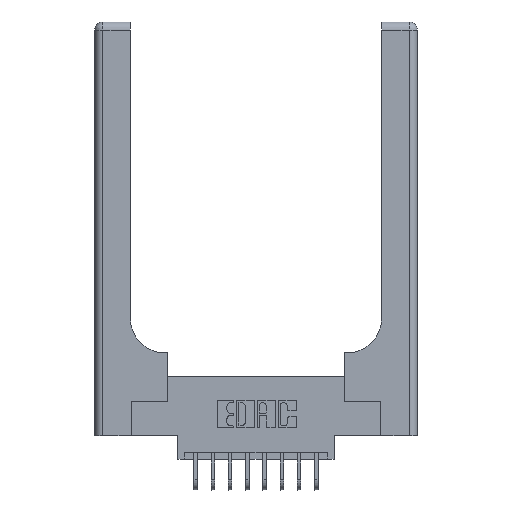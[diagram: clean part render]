
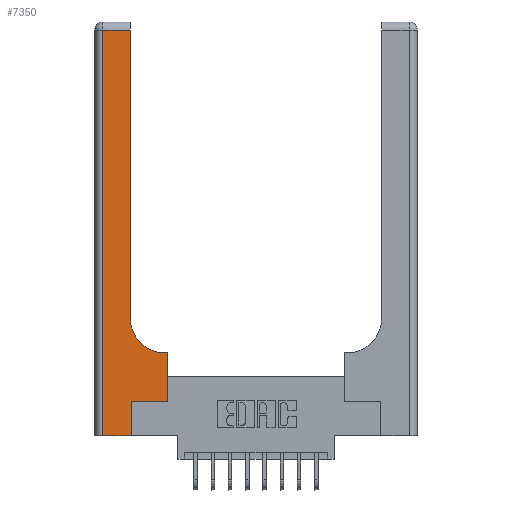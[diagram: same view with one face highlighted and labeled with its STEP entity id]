
A CAD part, top view. The second image highlights one B-rep face of the part: STEP entity #7350.
In plain terms, the highlighted planar face has unit normal (0, 0, 1).
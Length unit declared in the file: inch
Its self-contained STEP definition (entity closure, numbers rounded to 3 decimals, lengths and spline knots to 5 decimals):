
#139 = AXIS2_PLACEMENT_3D ( 'NONE', #10508, #4011, #13096 ) ;
#195 = LINE ( 'NONE', #4476, #13621 ) ;
#412 = CARTESIAN_POINT ( 'NONE',  ( 0.06, 3., 0.37 ) ) ;
#425 = ORIENTED_EDGE ( 'NONE', *, *, #13636, .T. ) ;
#870 = VECTOR ( 'NONE', #14672, 39.37008 ) ;
#946 = EDGE_CURVE ( 'NONE', #8027, #1399, #11583, .T. ) ;
#1140 = LINE ( 'NONE', #3094, #14382 ) ;
#1165 = CARTESIAN_POINT ( 'NONE',  ( 0.528, 0.25, 0.37 ) ) ;
#1182 = LINE ( 'NONE', #11846, #6109 ) ;
#1399 = VERTEX_POINT ( 'NONE', #14394 ) ;
#1741 = EDGE_CURVE ( 'NONE', #9085, #14748, #13734, .T. ) ;
#1754 = ORIENTED_EDGE ( 'NONE', *, *, #1741, .T. ) ;
#2352 = CARTESIAN_POINT ( 'NONE',  ( 0.528, 0.6, 0.37 ) ) ;
#2719 = PLANE ( 'NONE',  #139 ) ;
#2959 = CARTESIAN_POINT ( 'NONE',  ( 0.06, 2.94, 0.37 ) ) ;
#2977 = DIRECTION ( 'NONE',  ( -1., 0., 0. ) ) ;
#3094 = CARTESIAN_POINT ( 'NONE',  ( 0.26, 0.6, 0.37 ) ) ;
#3334 = ORIENTED_EDGE ( 'NONE', *, *, #13177, .T. ) ;
#3459 = CARTESIAN_POINT ( 'NONE',  ( 0.265, 0., 0.37 ) ) ;
#3474 = VERTEX_POINT ( 'NONE', #2959 ) ;
#3480 = EDGE_LOOP ( 'NONE', ( #13267, #8925, #3334, #16211, #7338, #14105, #1754, #425, #15475 ) ) ;
#3570 = CARTESIAN_POINT ( 'NONE',  ( 0.265, 0.25, 0.37 ) ) ;
#3919 = AXIS2_PLACEMENT_3D ( 'NONE', #12390, #7409, #16470 ) ;
#3924 = EDGE_CURVE ( 'NONE', #4167, #8027, #4488, .T. ) ;
#4011 = DIRECTION ( 'NONE',  ( 0., 0., -1. ) ) ;
#4067 = DIRECTION ( 'NONE',  ( 0., 1., 0. ) ) ;
#4167 = VERTEX_POINT ( 'NONE', #5222 ) ;
#4476 = CARTESIAN_POINT ( 'NONE',  ( 0., 2.94, 0.37 ) ) ;
#4488 = CIRCLE ( 'NONE', #3919, 0.25 ) ;
#4584 = VECTOR ( 'NONE', #5874, 39.37008 ) ;
#4842 = LINE ( 'NONE', #412, #16899 ) ;
#5222 = CARTESIAN_POINT ( 'NONE',  ( 0.51, 0.6, 0.37 ) ) ;
#5644 = DIRECTION ( 'NONE',  ( 0., -1., 0. ) ) ;
#5874 = DIRECTION ( 'NONE',  ( 1., 0., 0. ) ) ;
#6109 = VECTOR ( 'NONE', #4067, 39.37008 ) ;
#6215 = DIRECTION ( 'NONE',  ( -1., 0., 0. ) ) ;
#6442 = LINE ( 'NONE', #10901, #12468 ) ;
#6463 = CARTESIAN_POINT ( 'NONE',  ( 0.26, 0.85, 0.37 ) ) ;
#6642 = CARTESIAN_POINT ( 'NONE',  ( 0.06, 0., 0.37 ) ) ;
#6921 = FACE_OUTER_BOUND ( 'NONE', #3480, .T. ) ;
#6977 = CARTESIAN_POINT ( 'NONE',  ( 0.528, 0.25, 0.37 ) ) ;
#7338 = ORIENTED_EDGE ( 'NONE', *, *, #7373, .T. ) ;
#7350 = ADVANCED_FACE ( 'NONE', ( #6921 ), #2719, .F. ) ;
#7373 = EDGE_CURVE ( 'NONE', #14707, #9164, #1182, .T. ) ;
#7409 = DIRECTION ( 'NONE',  ( 0., 0., -1. ) ) ;
#7734 = EDGE_CURVE ( 'NONE', #9164, #9085, #16669, .T. ) ;
#8027 = VERTEX_POINT ( 'NONE', #6463 ) ;
#8482 = EDGE_CURVE ( 'NONE', #8859, #14707, #6442, .T. ) ;
#8859 = VERTEX_POINT ( 'NONE', #6642 ) ;
#8925 = ORIENTED_EDGE ( 'NONE', *, *, #11923, .T. ) ;
#9085 = VERTEX_POINT ( 'NONE', #6977 ) ;
#9164 = VERTEX_POINT ( 'NONE', #3570 ) ;
#10373 = CARTESIAN_POINT ( 'NONE',  ( 0.26, 3., 0.37 ) ) ;
#10508 = CARTESIAN_POINT ( 'NONE',  ( 0., 3., 0.37 ) ) ;
#10901 = CARTESIAN_POINT ( 'NONE',  ( 0., 0., 0.37 ) ) ;
#11173 = VECTOR ( 'NONE', #12941, 39.37008 ) ;
#11583 = LINE ( 'NONE', #10373, #11173 ) ;
#11846 = CARTESIAN_POINT ( 'NONE',  ( 0.265, 0., 0.37 ) ) ;
#11923 = EDGE_CURVE ( 'NONE', #1399, #3474, #195, .T. ) ;
#12390 = CARTESIAN_POINT ( 'NONE',  ( 0.51, 0.85, 0.37 ) ) ;
#12468 = VECTOR ( 'NONE', #13283, 39.37008 ) ;
#12941 = DIRECTION ( 'NONE',  ( 0., 1., 0. ) ) ;
#13096 = DIRECTION ( 'NONE',  ( -1., 0., 0. ) ) ;
#13177 = EDGE_CURVE ( 'NONE', #3474, #8859, #4842, .T. ) ;
#13267 = ORIENTED_EDGE ( 'NONE', *, *, #946, .T. ) ;
#13283 = DIRECTION ( 'NONE',  ( 1., 0., 0. ) ) ;
#13418 = CARTESIAN_POINT ( 'NONE',  ( 0.265, 0.25, 0.37 ) ) ;
#13621 = VECTOR ( 'NONE', #6215, 39.37008 ) ;
#13636 = EDGE_CURVE ( 'NONE', #14748, #4167, #1140, .T. ) ;
#13734 = LINE ( 'NONE', #1165, #870 ) ;
#14105 = ORIENTED_EDGE ( 'NONE', *, *, #7734, .T. ) ;
#14382 = VECTOR ( 'NONE', #2977, 39.37008 ) ;
#14394 = CARTESIAN_POINT ( 'NONE',  ( 0.26, 2.94, 0.37 ) ) ;
#14672 = DIRECTION ( 'NONE',  ( 0., 1., 0. ) ) ;
#14707 = VERTEX_POINT ( 'NONE', #3459 ) ;
#14748 = VERTEX_POINT ( 'NONE', #2352 ) ;
#15475 = ORIENTED_EDGE ( 'NONE', *, *, #3924, .T. ) ;
#16211 = ORIENTED_EDGE ( 'NONE', *, *, #8482, .T. ) ;
#16470 = DIRECTION ( 'NONE',  ( 1., 0., 0. ) ) ;
#16669 = LINE ( 'NONE', #13418, #4584 ) ;
#16899 = VECTOR ( 'NONE', #5644, 39.37008 ) ;
